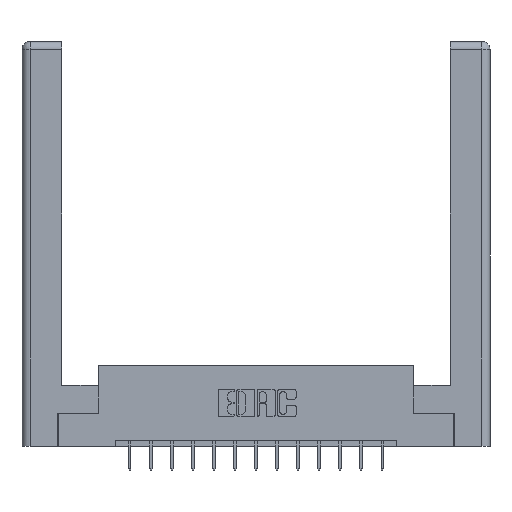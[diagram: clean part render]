
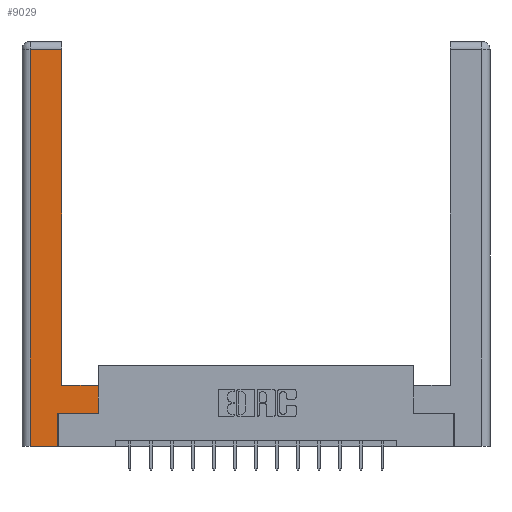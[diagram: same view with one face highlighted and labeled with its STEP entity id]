
A CAD part, top view. The second image highlights one B-rep face of the part: STEP entity #9029.
In plain terms, the highlighted planar face has unit normal (0, 0, 1).
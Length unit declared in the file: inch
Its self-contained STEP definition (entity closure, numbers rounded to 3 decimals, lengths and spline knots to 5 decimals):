
#81 = CARTESIAN_POINT ( 'NONE',  ( 0.295, 0.45, 0. ) ) ;
#362 = PLANE ( 'NONE',  #11965 ) ;
#563 = EDGE_CURVE ( 'NONE', #14278, #10031, #14940, .T. ) ;
#758 = VERTEX_POINT ( 'NONE', #13084 ) ;
#889 = CARTESIAN_POINT ( 'NONE',  ( 0.0615, 2.94, 0. ) ) ;
#1707 = EDGE_LOOP ( 'NONE', ( #13799, #7200, #15653, #11706, #10664, #10747, #4117, #10169 ) ) ;
#2329 = CARTESIAN_POINT ( 'NONE',  ( 0.565, 0.45, 0. ) ) ;
#2587 = LINE ( 'NONE', #889, #8537 ) ;
#2900 = EDGE_CURVE ( 'NONE', #12225, #13965, #2587, .T. ) ;
#2911 = DIRECTION ( 'NONE',  ( 0., 0., -1. ) ) ;
#2914 = CARTESIAN_POINT ( 'NONE',  ( 0.0615, 2.94, 0. ) ) ;
#3116 = VECTOR ( 'NONE', #9985, 39.37008 ) ;
#3440 = LINE ( 'NONE', #6613, #9831 ) ;
#3838 = CARTESIAN_POINT ( 'NONE',  ( 0.295, 0.45, 0. ) ) ;
#4117 = ORIENTED_EDGE ( 'NONE', *, *, #6490, .T. ) ;
#4151 = VECTOR ( 'NONE', #11281, 39.37008 ) ;
#5254 = DIRECTION ( 'NONE',  ( -1., 0., 0. ) ) ;
#6490 = EDGE_CURVE ( 'NONE', #8228, #14278, #12970, .T. ) ;
#6613 = CARTESIAN_POINT ( 'NONE',  ( 0.295, 3., 0. ) ) ;
#7200 = ORIENTED_EDGE ( 'NONE', *, *, #2900, .T. ) ;
#7278 = CARTESIAN_POINT ( 'NONE',  ( 0.265, 0., 0. ) ) ;
#7705 = LINE ( 'NONE', #14933, #4151 ) ;
#7926 = FACE_OUTER_BOUND ( 'NONE', #1707, .T. ) ;
#7950 = CARTESIAN_POINT ( 'NONE',  ( 0.565, 0.45, 0. ) ) ;
#8125 = CARTESIAN_POINT ( 'NONE',  ( 0.565, 0.245, 0. ) ) ;
#8228 = VERTEX_POINT ( 'NONE', #8125 ) ;
#8291 = LINE ( 'NONE', #7278, #3116 ) ;
#8537 = VECTOR ( 'NONE', #15080, 39.37008 ) ;
#9021 = CARTESIAN_POINT ( 'NONE',  ( 0.0615, 0., 0. ) ) ;
#9029 = ADVANCED_FACE ( 'NONE', ( #7926 ), #362, .F. ) ;
#9043 = DIRECTION ( 'NONE',  ( -1., 0., 0. ) ) ;
#9255 = VERTEX_POINT ( 'NONE', #9021 ) ;
#9266 = LINE ( 'NONE', #15883, #10868 ) ;
#9578 = EDGE_CURVE ( 'NONE', #758, #8228, #7705, .T. ) ;
#9831 = VECTOR ( 'NONE', #15381, 39.37008 ) ;
#9985 = DIRECTION ( 'NONE',  ( 1., 0., 0. ) ) ;
#10031 = VERTEX_POINT ( 'NONE', #3838 ) ;
#10169 = ORIENTED_EDGE ( 'NONE', *, *, #563, .T. ) ;
#10459 = CARTESIAN_POINT ( 'NONE',  ( 0., 0., 0. ) ) ;
#10664 = ORIENTED_EDGE ( 'NONE', *, *, #14455, .T. ) ;
#10688 = VERTEX_POINT ( 'NONE', #13485 ) ;
#10747 = ORIENTED_EDGE ( 'NONE', *, *, #9578, .T. ) ;
#10868 = VECTOR ( 'NONE', #14497, 39.37008 ) ;
#11011 = CARTESIAN_POINT ( 'NONE',  ( 0.295, 2.94, 0. ) ) ;
#11281 = DIRECTION ( 'NONE',  ( 1., 0., 0. ) ) ;
#11294 = VECTOR ( 'NONE', #14716, 39.37008 ) ;
#11388 = EDGE_CURVE ( 'NONE', #10031, #12225, #3440, .T. ) ;
#11522 = LINE ( 'NONE', #13371, #11294 ) ;
#11540 = VECTOR ( 'NONE', #5254, 39.37008 ) ;
#11706 = ORIENTED_EDGE ( 'NONE', *, *, #14007, .T. ) ;
#11965 = AXIS2_PLACEMENT_3D ( 'NONE', #10459, #2911, #9043 ) ;
#12225 = VERTEX_POINT ( 'NONE', #11011 ) ;
#12970 = LINE ( 'NONE', #2329, #15598 ) ;
#13084 = CARTESIAN_POINT ( 'NONE',  ( 0.265, 0.245, 0. ) ) ;
#13371 = CARTESIAN_POINT ( 'NONE',  ( 0.265, 0.245, 0. ) ) ;
#13485 = CARTESIAN_POINT ( 'NONE',  ( 0.265, 0., 0. ) ) ;
#13799 = ORIENTED_EDGE ( 'NONE', *, *, #11388, .T. ) ;
#13965 = VERTEX_POINT ( 'NONE', #2914 ) ;
#14007 = EDGE_CURVE ( 'NONE', #9255, #10688, #8291, .T. ) ;
#14278 = VERTEX_POINT ( 'NONE', #7950 ) ;
#14455 = EDGE_CURVE ( 'NONE', #10688, #758, #11522, .T. ) ;
#14497 = DIRECTION ( 'NONE',  ( 0., -1., 0. ) ) ;
#14716 = DIRECTION ( 'NONE',  ( 0., 1., 0. ) ) ;
#14933 = CARTESIAN_POINT ( 'NONE',  ( 0.565, 0.245, 0. ) ) ;
#14940 = LINE ( 'NONE', #81, #11540 ) ;
#15080 = DIRECTION ( 'NONE',  ( -1., 0., 0. ) ) ;
#15193 = DIRECTION ( 'NONE',  ( 0., 1., 0. ) ) ;
#15381 = DIRECTION ( 'NONE',  ( 0., 1., 0. ) ) ;
#15598 = VECTOR ( 'NONE', #15193, 39.37008 ) ;
#15653 = ORIENTED_EDGE ( 'NONE', *, *, #16006, .T. ) ;
#15883 = CARTESIAN_POINT ( 'NONE',  ( 0.0615, 0., 0. ) ) ;
#16006 = EDGE_CURVE ( 'NONE', #13965, #9255, #9266, .T. ) ;
